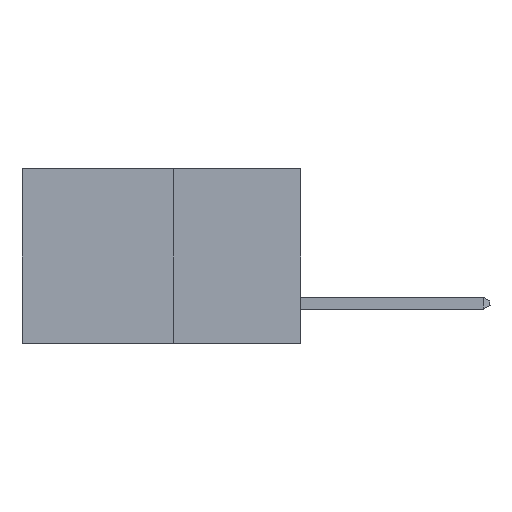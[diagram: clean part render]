
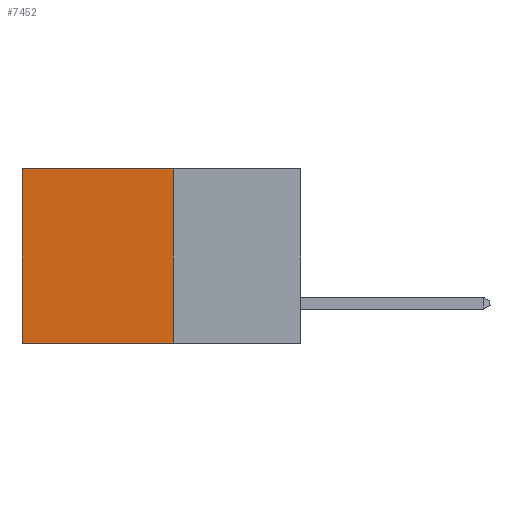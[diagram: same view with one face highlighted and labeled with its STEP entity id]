
A CAD part, left-side view. The second image highlights one B-rep face of the part: STEP entity #7452.
In plain terms, the highlighted planar face has unit normal (-1, 0, 0).
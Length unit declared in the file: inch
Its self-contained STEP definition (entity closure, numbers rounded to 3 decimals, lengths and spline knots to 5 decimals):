
#1554 = EDGE_CURVE ( 'NONE', #7970, #13464, #7781, .T. ) ;
#1764 = CARTESIAN_POINT ( 'NONE',  ( 0.277, 0.27, -0.37 ) ) ;
#2280 = CARTESIAN_POINT ( 'NONE',  ( 0.277, 0.27, 0. ) ) ;
#2587 = EDGE_CURVE ( 'NONE', #7970, #13993, #13135, .T. ) ;
#3670 = AXIS2_PLACEMENT_3D ( 'NONE', #11252, #3798, #12516 ) ;
#3798 = DIRECTION ( 'NONE',  ( 1., 0., 0. ) ) ;
#4466 = ORIENTED_EDGE ( 'NONE', *, *, #5741, .T. ) ;
#4555 = ORIENTED_EDGE ( 'NONE', *, *, #9746, .F. ) ;
#4707 = ORIENTED_EDGE ( 'NONE', *, *, #1554, .F. ) ;
#4777 = ORIENTED_EDGE ( 'NONE', *, *, #2587, .T. ) ;
#5183 = LINE ( 'NONE', #11087, #14325 ) ;
#5741 = EDGE_CURVE ( 'NONE', #13993, #7394, #13439, .T. ) ;
#5788 = CARTESIAN_POINT ( 'NONE',  ( 0.277, 0.27, 0. ) ) ;
#5851 = DIRECTION ( 'NONE',  ( 0., 1., 0. ) ) ;
#6836 = EDGE_LOOP ( 'NONE', ( #4466, #4555, #4707, #4777 ) ) ;
#7394 = VERTEX_POINT ( 'NONE', #14897 ) ;
#7452 = ADVANCED_FACE ( 'NONE', ( #14398 ), #8821, .F. ) ;
#7781 = LINE ( 'NONE', #13887, #13972 ) ;
#7970 = VERTEX_POINT ( 'NONE', #2280 ) ;
#8278 = DIRECTION ( 'NONE',  ( 0., 0., -1. ) ) ;
#8821 = PLANE ( 'NONE',  #3670 ) ;
#9746 = EDGE_CURVE ( 'NONE', #13464, #7394, #5183, .T. ) ;
#9772 = VECTOR ( 'NONE', #8278, 39.37008 ) ;
#11087 = CARTESIAN_POINT ( 'NONE',  ( 0.277, 0.27, -0.37 ) ) ;
#11252 = CARTESIAN_POINT ( 'NONE',  ( 0.277, 0.27, -0.37 ) ) ;
#12355 = DIRECTION ( 'NONE',  ( 0., 1., 0. ) ) ;
#12516 = DIRECTION ( 'NONE',  ( 0., 0., -1. ) ) ;
#13135 = LINE ( 'NONE', #5788, #13924 ) ;
#13439 = LINE ( 'NONE', #14410, #9772 ) ;
#13464 = VERTEX_POINT ( 'NONE', #1764 ) ;
#13825 = DIRECTION ( 'NONE',  ( 0., 0., -1. ) ) ;
#13887 = CARTESIAN_POINT ( 'NONE',  ( 0.277, 0.27, -0.37 ) ) ;
#13924 = VECTOR ( 'NONE', #5851, 39.37008 ) ;
#13972 = VECTOR ( 'NONE', #13825, 39.37008 ) ;
#13993 = VERTEX_POINT ( 'NONE', #15076 ) ;
#14325 = VECTOR ( 'NONE', #12355, 39.37008 ) ;
#14398 = FACE_OUTER_BOUND ( 'NONE', #6836, .T. ) ;
#14410 = CARTESIAN_POINT ( 'NONE',  ( 0.277, 0.59, -0.37 ) ) ;
#14897 = CARTESIAN_POINT ( 'NONE',  ( 0.277, 0.59, -0.37 ) ) ;
#15076 = CARTESIAN_POINT ( 'NONE',  ( 0.277, 0.59, 0. ) ) ;
